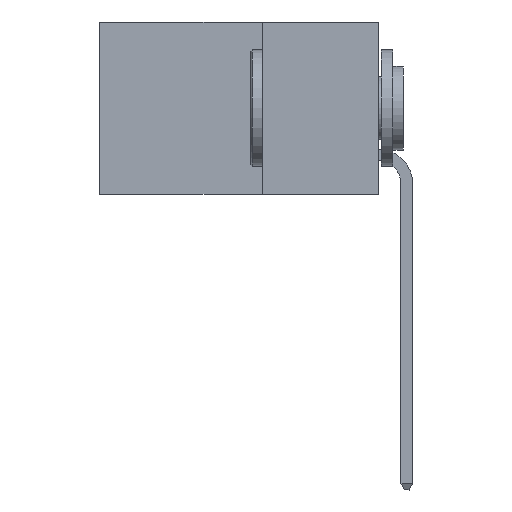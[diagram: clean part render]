
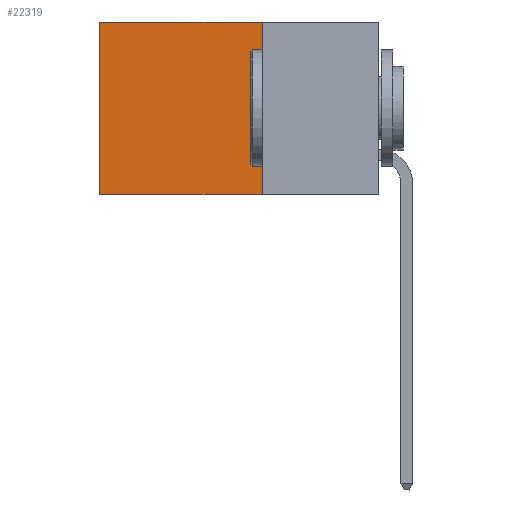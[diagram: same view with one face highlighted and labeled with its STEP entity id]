
A CAD part, left-side view. The second image highlights one B-rep face of the part: STEP entity #22319.
In plain terms, the highlighted planar face has unit normal (-1, 0, 0).
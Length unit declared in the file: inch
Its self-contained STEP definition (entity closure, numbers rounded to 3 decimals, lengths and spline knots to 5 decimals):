
#103 = EDGE_CURVE ( 'NONE', #5594, #18292, #6232, .T. ) ;
#322 = VECTOR ( 'NONE', #11631, 39.37008 ) ;
#1785 = EDGE_CURVE ( 'NONE', #14212, #18292, #25281, .T. ) ;
#1899 = EDGE_LOOP ( 'NONE', ( #8921, #27591, #9764, #15853 ) ) ;
#2295 = DIRECTION ( 'NONE',  ( 1., 0., 0. ) ) ;
#3627 = CARTESIAN_POINT ( 'NONE',  ( 0.298, 0.25, 0. ) ) ;
#4390 = CARTESIAN_POINT ( 'NONE',  ( 0.298, 0.25, -0.37 ) ) ;
#5352 = VECTOR ( 'NONE', #27558, 39.37008 ) ;
#5594 = VERTEX_POINT ( 'NONE', #10980 ) ;
#5915 = FACE_OUTER_BOUND ( 'NONE', #1899, .T. ) ;
#6232 = LINE ( 'NONE', #4390, #322 ) ;
#7648 = VECTOR ( 'NONE', #18985, 39.37008 ) ;
#8580 = VECTOR ( 'NONE', #19447, 39.37008 ) ;
#8921 = ORIENTED_EDGE ( 'NONE', *, *, #1785, .T. ) ;
#9764 = ORIENTED_EDGE ( 'NONE', *, *, #12476, .F. ) ;
#10980 = CARTESIAN_POINT ( 'NONE',  ( 0.298, 0.25, -0.37 ) ) ;
#11631 = DIRECTION ( 'NONE',  ( 0., 1., 0. ) ) ;
#12476 = EDGE_CURVE ( 'NONE', #20552, #5594, #16982, .T. ) ;
#14212 = VERTEX_POINT ( 'NONE', #18151 ) ;
#14403 = CARTESIAN_POINT ( 'NONE',  ( 0.298, 0.25, 0. ) ) ;
#15853 = ORIENTED_EDGE ( 'NONE', *, *, #16311, .T. ) ;
#16311 = EDGE_CURVE ( 'NONE', #20552, #14212, #22986, .T. ) ;
#16982 = LINE ( 'NONE', #27474, #5352 ) ;
#17528 = AXIS2_PLACEMENT_3D ( 'NONE', #19776, #2295, #17658 ) ;
#17658 = DIRECTION ( 'NONE',  ( 0., 0., -1. ) ) ;
#18151 = CARTESIAN_POINT ( 'NONE',  ( 0.298, 0.6, 0. ) ) ;
#18292 = VERTEX_POINT ( 'NONE', #24024 ) ;
#18555 = CARTESIAN_POINT ( 'NONE',  ( 0.298, 0.6, 0. ) ) ;
#18985 = DIRECTION ( 'NONE',  ( 0., 1., 0. ) ) ;
#19447 = DIRECTION ( 'NONE',  ( 0., 0., -1. ) ) ;
#19776 = CARTESIAN_POINT ( 'NONE',  ( 0.298, 0.25, 0. ) ) ;
#20552 = VERTEX_POINT ( 'NONE', #14403 ) ;
#22319 = ADVANCED_FACE ( 'NONE', ( #5915 ), #24118, .F. ) ;
#22986 = LINE ( 'NONE', #3627, #7648 ) ;
#24024 = CARTESIAN_POINT ( 'NONE',  ( 0.298, 0.6, -0.37 ) ) ;
#24118 = PLANE ( 'NONE',  #17528 ) ;
#25281 = LINE ( 'NONE', #18555, #8580 ) ;
#27474 = CARTESIAN_POINT ( 'NONE',  ( 0.298, 0.25, 0. ) ) ;
#27558 = DIRECTION ( 'NONE',  ( 0., 0., -1. ) ) ;
#27591 = ORIENTED_EDGE ( 'NONE', *, *, #103, .F. ) ;
